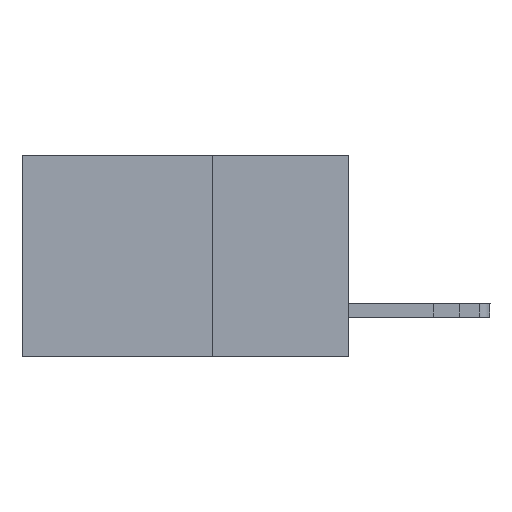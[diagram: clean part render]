
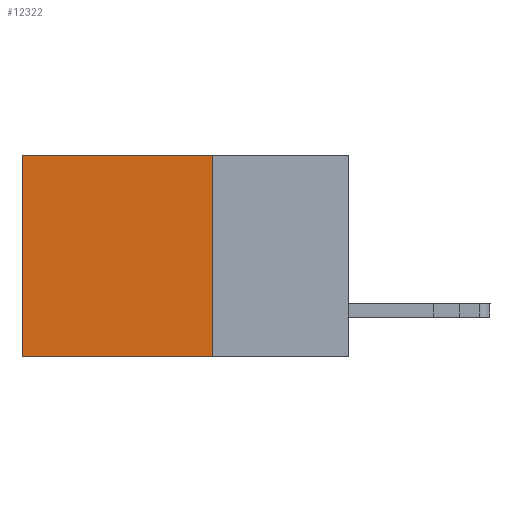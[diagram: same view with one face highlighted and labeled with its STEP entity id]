
A CAD part, left-side view. The second image highlights one B-rep face of the part: STEP entity #12322.
In plain terms, the highlighted planar face has unit normal (-1, 0, 0).
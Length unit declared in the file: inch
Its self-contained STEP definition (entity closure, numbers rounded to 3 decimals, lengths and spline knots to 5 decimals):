
#187 = EDGE_CURVE ( 'NONE', #10994, #19976, #11137, .T. ) ;
#997 = EDGE_CURVE ( 'NONE', #19976, #9836, #15598, .T. ) ;
#1184 = AXIS2_PLACEMENT_3D ( 'NONE', #12948, #5006, #9868 ) ;
#1266 = CARTESIAN_POINT ( 'NONE',  ( 0.2615, 0.25, -0.37 ) ) ;
#1349 = CARTESIAN_POINT ( 'NONE',  ( 0.2615, 0.6, 0. ) ) ;
#1887 = VECTOR ( 'NONE', #15744, 39.37008 ) ;
#2528 = EDGE_LOOP ( 'NONE', ( #15155, #12679, #17416, #13116 ) ) ;
#3564 = FACE_OUTER_BOUND ( 'NONE', #2528, .T. ) ;
#3999 = EDGE_CURVE ( 'NONE', #17563, #9836, #6433, .T. ) ;
#5003 = CARTESIAN_POINT ( 'NONE',  ( 0.2615, 0.6, -0.37 ) ) ;
#5006 = DIRECTION ( 'NONE',  ( 1., 0., 0. ) ) ;
#5723 = CARTESIAN_POINT ( 'NONE',  ( 0.2615, 0.25, 0. ) ) ;
#6123 = DIRECTION ( 'NONE',  ( 0., 1., 0. ) ) ;
#6433 = LINE ( 'NONE', #18953, #13122 ) ;
#6769 = PLANE ( 'NONE',  #1184 ) ;
#9488 = CARTESIAN_POINT ( 'NONE',  ( 0.2615, 0.25, -0.37 ) ) ;
#9836 = VERTEX_POINT ( 'NONE', #5003 ) ;
#9868 = DIRECTION ( 'NONE',  ( 0., 0., -1. ) ) ;
#10994 = VERTEX_POINT ( 'NONE', #11413 ) ;
#11137 = LINE ( 'NONE', #9488, #1887 ) ;
#11413 = CARTESIAN_POINT ( 'NONE',  ( 0.2615, 0.25, 0. ) ) ;
#12322 = ADVANCED_FACE ( 'NONE', ( #3564 ), #6769, .F. ) ;
#12456 = EDGE_CURVE ( 'NONE', #10994, #17563, #19488, .T. ) ;
#12679 = ORIENTED_EDGE ( 'NONE', *, *, #997, .F. ) ;
#12712 = CARTESIAN_POINT ( 'NONE',  ( 0.2615, 0.25, -0.37 ) ) ;
#12718 = DIRECTION ( 'NONE',  ( 0., 0., -1. ) ) ;
#12948 = CARTESIAN_POINT ( 'NONE',  ( 0.2615, 0.25, -0.37 ) ) ;
#13116 = ORIENTED_EDGE ( 'NONE', *, *, #12456, .T. ) ;
#13122 = VECTOR ( 'NONE', #12718, 39.37008 ) ;
#14970 = VECTOR ( 'NONE', #16513, 39.37008 ) ;
#15155 = ORIENTED_EDGE ( 'NONE', *, *, #3999, .T. ) ;
#15598 = LINE ( 'NONE', #12712, #16666 ) ;
#15744 = DIRECTION ( 'NONE',  ( 0., 0., -1. ) ) ;
#16513 = DIRECTION ( 'NONE',  ( 0., 1., 0. ) ) ;
#16666 = VECTOR ( 'NONE', #6123, 39.37008 ) ;
#17416 = ORIENTED_EDGE ( 'NONE', *, *, #187, .F. ) ;
#17563 = VERTEX_POINT ( 'NONE', #1349 ) ;
#18953 = CARTESIAN_POINT ( 'NONE',  ( 0.2615, 0.6, -0.37 ) ) ;
#19488 = LINE ( 'NONE', #5723, #14970 ) ;
#19976 = VERTEX_POINT ( 'NONE', #1266 ) ;
